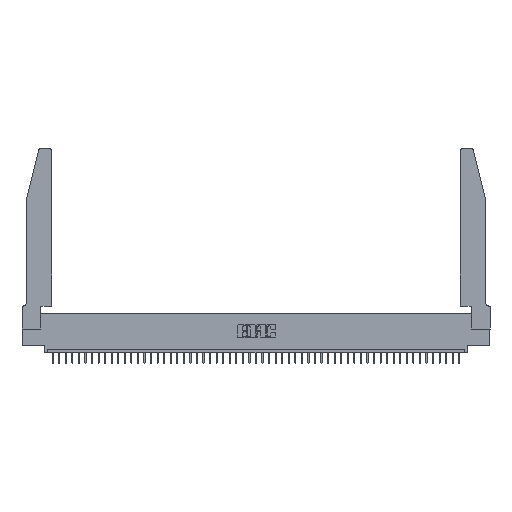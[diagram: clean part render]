
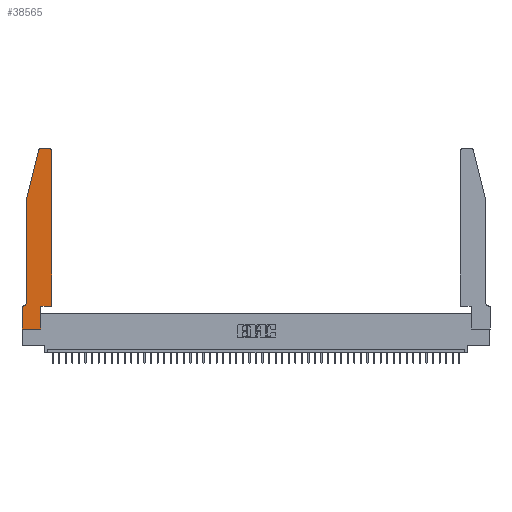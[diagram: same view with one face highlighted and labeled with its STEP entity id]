
A CAD part, top view. The second image highlights one B-rep face of the part: STEP entity #38565.
In plain terms, the highlighted planar face has unit normal (0, 0, 1).
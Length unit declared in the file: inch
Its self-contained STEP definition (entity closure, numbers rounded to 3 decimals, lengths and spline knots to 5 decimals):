
#819 = CARTESIAN_POINT ( 'NONE',  ( 0.2865, 0.35, 0.37 ) ) ;
#1431 = DIRECTION ( 'NONE',  ( 0., 0., 1. ) ) ;
#2141 = AXIS2_PLACEMENT_3D ( 'NONE', #9338, #20926, #24781 ) ;
#3712 = DIRECTION ( 'NONE',  ( -1., 0., 0. ) ) ;
#4256 = CARTESIAN_POINT ( 'NONE',  ( 0.4205, 2.75, 0.37 ) ) ;
#4876 = DIRECTION ( 'NONE',  ( 0., 0., 1. ) ) ;
#5688 = DIRECTION ( 'NONE',  ( -1., 0., 0. ) ) ;
#5836 = EDGE_CURVE ( 'NONE', #13979, #20223, #39087, .T. ) ;
#7107 = DIRECTION ( 'NONE',  ( -0.239, -0.971, 0. ) ) ;
#8033 = EDGE_LOOP ( 'NONE', ( #35172, #38126, #22997, #33671, #28231, #29537, #45173, #15679, #39279, #31077, #10825, #30660 ) ) ;
#8539 = DIRECTION ( 'NONE',  ( 1., 0., 0. ) ) ;
#9338 = CARTESIAN_POINT ( 'NONE',  ( 0.0055, 0.42, 0.37 ) ) ;
#9886 = VERTEX_POINT ( 'NONE', #30062 ) ;
#10825 = ORIENTED_EDGE ( 'NONE', *, *, #24829, .T. ) ;
#11740 = VERTEX_POINT ( 'NONE', #36055 ) ;
#12969 = CARTESIAN_POINT ( 'NONE',  ( 0., 0., 0.37 ) ) ;
#13102 = DIRECTION ( 'NONE',  ( 0., -1., 0. ) ) ;
#13517 = PLANE ( 'NONE',  #46264 ) ;
#13979 = VERTEX_POINT ( 'NONE', #20492 ) ;
#14463 = DIRECTION ( 'NONE',  ( 0., 1., 0. ) ) ;
#14923 = LINE ( 'NONE', #43565, #32215 ) ;
#15536 = CARTESIAN_POINT ( 'NONE',  ( 0.2865, 0., 0.37 ) ) ;
#15565 = LINE ( 'NONE', #12969, #42529 ) ;
#15679 = ORIENTED_EDGE ( 'NONE', *, *, #19875, .T. ) ;
#15707 = EDGE_CURVE ( 'NONE', #34347, #45064, #40745, .T. ) ;
#16875 = DIRECTION ( 'NONE',  ( 0., 1., 0. ) ) ;
#17169 = LINE ( 'NONE', #819, #27261 ) ;
#18559 = VECTOR ( 'NONE', #7107, 39.37008 ) ;
#18669 = CARTESIAN_POINT ( 'NONE',  ( 0.0755, 2., 0.37 ) ) ;
#19875 = EDGE_CURVE ( 'NONE', #9886, #28396, #43309, .T. ) ;
#20143 = LINE ( 'NONE', #27726, #21974 ) ;
#20149 = CARTESIAN_POINT ( 'NONE',  ( 0., 0., 0.37 ) ) ;
#20223 = VERTEX_POINT ( 'NONE', #35847 ) ;
#20492 = CARTESIAN_POINT ( 'NONE',  ( 0.2865, 0.35, 0.37 ) ) ;
#20779 = CARTESIAN_POINT ( 'NONE',  ( 0.0755, 0.35, 0.37 ) ) ;
#20926 = DIRECTION ( 'NONE',  ( 0., 0., -1. ) ) ;
#21596 = LINE ( 'NONE', #20779, #33542 ) ;
#21974 = VECTOR ( 'NONE', #16875, 39.37008 ) ;
#22807 = VERTEX_POINT ( 'NONE', #38792 ) ;
#22997 = ORIENTED_EDGE ( 'NONE', *, *, #45542, .T. ) ;
#24366 = DIRECTION ( 'NONE',  ( 0., -1., 0. ) ) ;
#24494 = VERTEX_POINT ( 'NONE', #31071 ) ;
#24781 = DIRECTION ( 'NONE',  ( -1., 0., 0. ) ) ;
#24829 = EDGE_CURVE ( 'NONE', #20223, #34347, #20143, .T. ) ;
#25127 = EDGE_CURVE ( 'NONE', #28396, #13979, #17169, .T. ) ;
#25266 = AXIS2_PLACEMENT_3D ( 'NONE', #40315, #4876, #26055 ) ;
#25594 = LINE ( 'NONE', #46210, #28551 ) ;
#26055 = DIRECTION ( 'NONE',  ( 1., 0., 0. ) ) ;
#26397 = VERTEX_POINT ( 'NONE', #45229 ) ;
#27261 = VECTOR ( 'NONE', #14463, 39.37008 ) ;
#27440 = VERTEX_POINT ( 'NONE', #31818 ) ;
#27726 = CARTESIAN_POINT ( 'NONE',  ( 0.4505, 0.35, 0.37 ) ) ;
#28231 = ORIENTED_EDGE ( 'NONE', *, *, #30768, .T. ) ;
#28396 = VERTEX_POINT ( 'NONE', #15536 ) ;
#28551 = VECTOR ( 'NONE', #3712, 39.37008 ) ;
#29537 = ORIENTED_EDGE ( 'NONE', *, *, #46850, .T. ) ;
#30062 = CARTESIAN_POINT ( 'NONE',  ( 0., 0., 0.37 ) ) ;
#30636 = EDGE_CURVE ( 'NONE', #42710, #22807, #48233, .T. ) ;
#30660 = ORIENTED_EDGE ( 'NONE', *, *, #15707, .T. ) ;
#30706 = VECTOR ( 'NONE', #8539, 39.37008 ) ;
#30768 = EDGE_CURVE ( 'NONE', #26397, #27440, #45852, .T. ) ;
#31071 = CARTESIAN_POINT ( 'NONE',  ( 0.0755, 2., 0.37 ) ) ;
#31077 = ORIENTED_EDGE ( 'NONE', *, *, #5836, .T. ) ;
#31818 = CARTESIAN_POINT ( 'NONE',  ( 0.0055, 0.35, 0.37 ) ) ;
#32069 = DIRECTION ( 'NONE',  ( 1., 0., 0. ) ) ;
#32215 = VECTOR ( 'NONE', #13102, 39.37008 ) ;
#33542 = VECTOR ( 'NONE', #5688, 39.37008 ) ;
#33671 = ORIENTED_EDGE ( 'NONE', *, *, #36024, .T. ) ;
#34347 = VERTEX_POINT ( 'NONE', #38557 ) ;
#35172 = ORIENTED_EDGE ( 'NONE', *, *, #43328, .T. ) ;
#35407 = EDGE_CURVE ( 'NONE', #11740, #9886, #15565, .T. ) ;
#35776 = CARTESIAN_POINT ( 'NONE',  ( 0.284, 2.72, 0.37 ) ) ;
#35847 = CARTESIAN_POINT ( 'NONE',  ( 0.4505, 0.35, 0.37 ) ) ;
#36024 = EDGE_CURVE ( 'NONE', #24494, #26397, #14923, .T. ) ;
#36055 = CARTESIAN_POINT ( 'NONE',  ( 0., 0.35, 0.37 ) ) ;
#36708 = VECTOR ( 'NONE', #47348, 39.37008 ) ;
#37080 = LINE ( 'NONE', #18669, #18559 ) ;
#38126 = ORIENTED_EDGE ( 'NONE', *, *, #30636, .T. ) ;
#38557 = CARTESIAN_POINT ( 'NONE',  ( 0.4505, 2.72, 0.37 ) ) ;
#38565 = ADVANCED_FACE ( 'NONE', ( #41000 ), #13517, .T. ) ;
#38792 = CARTESIAN_POINT ( 'NONE',  ( 0.25487, 2.72718, 0.37 ) ) ;
#38969 = DIRECTION ( 'NONE',  ( 1., 0., 0. ) ) ;
#39087 = LINE ( 'NONE', #39159, #36708 ) ;
#39159 = CARTESIAN_POINT ( 'NONE',  ( 0.4505, 0.35, 0.37 ) ) ;
#39279 = ORIENTED_EDGE ( 'NONE', *, *, #25127, .T. ) ;
#40148 = CARTESIAN_POINT ( 'NONE',  ( 0., 0.35, 0.37 ) ) ;
#40315 = CARTESIAN_POINT ( 'NONE',  ( 0.4205, 2.72, 0.37 ) ) ;
#40745 = CIRCLE ( 'NONE', #25266, 0.03 ) ;
#41000 = FACE_OUTER_BOUND ( 'NONE', #8033, .T. ) ;
#42529 = VECTOR ( 'NONE', #24366, 39.37008 ) ;
#42710 = VERTEX_POINT ( 'NONE', #44951 ) ;
#43309 = LINE ( 'NONE', #20149, #30706 ) ;
#43328 = EDGE_CURVE ( 'NONE', #45064, #42710, #25594, .T. ) ;
#43565 = CARTESIAN_POINT ( 'NONE',  ( 0.0755, 2., 0.37 ) ) ;
#44457 = AXIS2_PLACEMENT_3D ( 'NONE', #35776, #47011, #38969 ) ;
#44951 = CARTESIAN_POINT ( 'NONE',  ( 0.284, 2.75, 0.37 ) ) ;
#45064 = VERTEX_POINT ( 'NONE', #4256 ) ;
#45173 = ORIENTED_EDGE ( 'NONE', *, *, #35407, .T. ) ;
#45229 = CARTESIAN_POINT ( 'NONE',  ( 0.0755, 0.42, 0.37 ) ) ;
#45542 = EDGE_CURVE ( 'NONE', #22807, #24494, #37080, .T. ) ;
#45852 = CIRCLE ( 'NONE', #2141, 0.07 ) ;
#46210 = CARTESIAN_POINT ( 'NONE',  ( 0.2605, 2.75, 0.37 ) ) ;
#46264 = AXIS2_PLACEMENT_3D ( 'NONE', #40148, #1431, #32069 ) ;
#46850 = EDGE_CURVE ( 'NONE', #27440, #11740, #21596, .T. ) ;
#47011 = DIRECTION ( 'NONE',  ( 0., 0., 1. ) ) ;
#47348 = DIRECTION ( 'NONE',  ( 1., 0., 0. ) ) ;
#48233 = CIRCLE ( 'NONE', #44457, 0.03 ) ;
